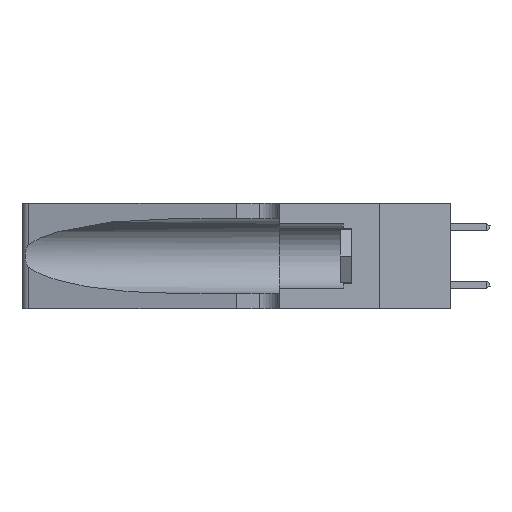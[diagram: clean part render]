
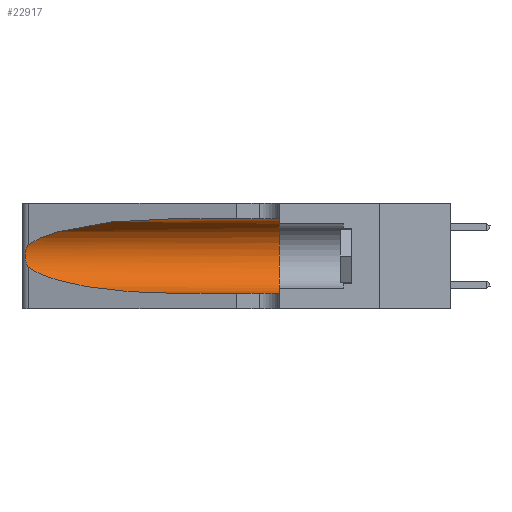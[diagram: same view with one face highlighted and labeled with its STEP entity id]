
A CAD part, left-side view. The second image highlights one B-rep face of the part: STEP entity #22917.
In plain terms, the highlighted cylindrical face has radius 3.308 mm (diameter 6.617 mm), a partial arc.
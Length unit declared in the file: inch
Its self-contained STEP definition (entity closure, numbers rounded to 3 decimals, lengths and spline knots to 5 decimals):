
#261 = AXIS2_PLACEMENT_3D ( 'NONE', #25124, #6758, #11429 ) ;
#1364 = DIRECTION ( 'NONE',  ( 0., -1., 0. ) ) ;
#1987 = CARTESIAN_POINT ( 'NONE',  ( 0.25487, 1.22718, 0.14631 ) ) ;
#2137 = CARTESIAN_POINT ( 'NONE',  ( 0.25639, 1.23184, 0.21858 ) ) ;
#2573 = ORIENTED_EDGE ( 'NONE', *, *, #3771, .T. ) ;
#2584 = CARTESIAN_POINT ( 'NONE',  ( 0.1305, 0.35, 0.05475 ) ) ;
#3664 = VERTEX_POINT ( 'NONE', #27870 ) ;
#3771 = EDGE_CURVE ( 'NONE', #14940, #25834, #26094, .T. ) ;
#3923 = CARTESIAN_POINT ( 'NONE',  ( 0.25487, 1.22718, 0.14631 ) ) ;
#4180 = AXIS2_PLACEMENT_3D ( 'NONE', #6070, #22220, #8388 ) ;
#4479 = CARTESIAN_POINT ( 'NONE',  ( 0.25854, 1.2359, 0.20912 ) ) ;
#4902 = CYLINDRICAL_SURFACE ( 'NONE', #261, 0.13025 ) ;
#5073 = CIRCLE ( 'NONE', #4180, 0.13025 ) ;
#5121 = CARTESIAN_POINT ( 'NONE',  ( 0.18966, 0.96281, 0.31525 ) ) ;
#5540 = ORIENTED_EDGE ( 'NONE', *, *, #24646, .F. ) ;
#6070 = CARTESIAN_POINT ( 'NONE',  ( 0.1305, 0.35, 0.185 ) ) ;
#6091 = B_SPLINE_CURVE_WITH_KNOTS ( 'NONE', 3,
 ( #25230, #13781, #2137, #18386, #4479, #20699, #6861, #23013, #9196, #25334, #11536, #27645, #13876, #29940 ),
 .UNSPECIFIED., .F., .F.,
 ( 4, 2, 2, 2, 2, 2, 4 ),
 ( 0., 0.00027, 0.00053, 0.00107, 0.0016, 0.00187, 0.00214 ),
 .UNSPECIFIED. ) ;
#6699 = EDGE_LOOP ( 'NONE', ( #2573, #14979, #21804, #27936, #10268, #5540 ) ) ;
#6758 = DIRECTION ( 'NONE',  ( 0., -1., 0. ) ) ;
#6861 = CARTESIAN_POINT ( 'NONE',  ( 0.26075, 1.23896, 0.19203 ) ) ;
#7002 = VECTOR ( 'NONE', #1364, 39.37008 ) ;
#8388 = DIRECTION ( 'NONE',  ( 0., 0., 1. ) ) ;
#8605 = VECTOR ( 'NONE', #23226, 39.37008 ) ;
#9196 = CARTESIAN_POINT ( 'NONE',  ( 0.26017, 1.23833, 0.17102 ) ) ;
#9337 = LINE ( 'NONE', #11652, #8605 ) ;
#9818 = CARTESIAN_POINT ( 'NONE',  ( 0.25487, 1.22718, 0.22369 ) ) ;
#10268 = ORIENTED_EDGE ( 'NONE', *, *, #13147, .F. ) ;
#11429 = DIRECTION ( 'NONE',  ( 0., 0., -1. ) ) ;
#11536 = CARTESIAN_POINT ( 'NONE',  ( 0.25789, 1.23486, 0.15765 ) ) ;
#11652 = CARTESIAN_POINT ( 'NONE',  ( 0.1305, 1.61858, 0.05475 ) ) ;
#12064 = CARTESIAN_POINT ( 'NONE',  ( 0.2373, 1.15595, 0.28018 ) ) ;
#12379 = CARTESIAN_POINT ( 'NONE',  ( 0.1305, 0.72297, 0.31525 ) ) ;
#13147 = EDGE_CURVE ( 'NONE', #3664, #26229, #5073, .T. ) ;
#13216 = CARTESIAN_POINT ( 'NONE',  ( 0.1305, 0.72297, 0.05475 ) ) ;
#13353 = EDGE_CURVE ( 'NONE', #25834, #23560, #6091, .T. ) ;
#13781 = CARTESIAN_POINT ( 'NONE',  ( 0.25555, 1.22994, 0.2215 ) ) ;
#13876 = CARTESIAN_POINT ( 'NONE',  ( 0.25555, 1.22993, 0.14849 ) ) ;
#14471 = VERTEX_POINT ( 'NONE', #13216 ) ;
#14940 = VERTEX_POINT ( 'NONE', #12379 ) ;
#14979 = ORIENTED_EDGE ( 'NONE', *, *, #13353, .T. ) ;
#15537 = CARTESIAN_POINT ( 'NONE',  ( 0.2373, 1.15595, 0.08982 ) ) ;
#15634 = CARTESIAN_POINT ( 'NONE',  ( 0.1305, 0.72297, 0.05475 ) ) ;
#18386 = CARTESIAN_POINT ( 'NONE',  ( 0.25787, 1.23484, 0.2124 ) ) ;
#19450 = CARTESIAN_POINT ( 'NONE',  ( 0.25487, 1.22718, 0.22369 ) ) ;
#20699 = CARTESIAN_POINT ( 'NONE',  ( 0.26018, 1.23835, 0.19895 ) ) ;
#21577 = EDGE_CURVE ( 'NONE', #23560, #14471, #28286, .T. ) ;
#21804 = ORIENTED_EDGE ( 'NONE', *, *, #21577, .T. ) ;
#22220 = DIRECTION ( 'NONE',  ( 0., 1., 0. ) ) ;
#22361 = EDGE_CURVE ( 'NONE', #14471, #26229, #9337, .T. ) ;
#22917 = ADVANCED_FACE ( 'NONE', ( #23356 ), #4902, .F. ) ;
#23013 = CARTESIAN_POINT ( 'NONE',  ( 0.26075, 1.23896, 0.178 ) ) ;
#23226 = DIRECTION ( 'NONE',  ( 0., -1., 0. ) ) ;
#23356 = FACE_OUTER_BOUND ( 'NONE', #6699, .T. ) ;
#23560 = VERTEX_POINT ( 'NONE', #1987 ) ;
#23621 = CARTESIAN_POINT ( 'NONE',  ( 0.1305, 0.72297, 0.31525 ) ) ;
#24646 = EDGE_CURVE ( 'NONE', #14940, #3664, #26139, .T. ) ;
#25124 = CARTESIAN_POINT ( 'NONE',  ( 0.1305, 1.61858, 0.185 ) ) ;
#25230 = CARTESIAN_POINT ( 'NONE',  ( 0.25487, 1.22718, 0.22369 ) ) ;
#25334 = CARTESIAN_POINT ( 'NONE',  ( 0.25856, 1.23593, 0.16098 ) ) ;
#25834 = VERTEX_POINT ( 'NONE', #19450 ) ;
#26094 =( BOUNDED_CURVE ( )  B_SPLINE_CURVE ( 3, ( #23621, #5121, #12064, #9818 ),
 .UNSPECIFIED., .F., .F. ) 
 B_SPLINE_CURVE_WITH_KNOTS ( ( 4, 4 ),
 ( 1.5708, 2.84003 ),
 .UNSPECIFIED. ) 
 CURVE ( )  GEOMETRIC_REPRESENTATION_ITEM ( )  RATIONAL_B_SPLINE_CURVE ( ( 1., 0.87, 0.87, 1. ) ) 
 REPRESENTATION_ITEM ( '' )  );
#26139 = LINE ( 'NONE', #28550, #7002 ) ;
#26229 = VERTEX_POINT ( 'NONE', #2584 ) ;
#27645 = CARTESIAN_POINT ( 'NONE',  ( 0.25639, 1.23186, 0.15144 ) ) ;
#27870 = CARTESIAN_POINT ( 'NONE',  ( 0.1305, 0.35, 0.31525 ) ) ;
#27936 = ORIENTED_EDGE ( 'NONE', *, *, #22361, .T. ) ;
#28286 =( BOUNDED_CURVE ( )  B_SPLINE_CURVE ( 3, ( #3923, #15537, #29387, #15634 ),
 .UNSPECIFIED., .F., .T. ) 
 B_SPLINE_CURVE_WITH_KNOTS ( ( 4, 4 ),
 ( 3.44316, 4.71239 ),
 .UNSPECIFIED. ) 
 CURVE ( )  GEOMETRIC_REPRESENTATION_ITEM ( )  RATIONAL_B_SPLINE_CURVE ( ( 1., 0.87, 0.87, 1. ) ) 
 REPRESENTATION_ITEM ( '' )  );
#28550 = CARTESIAN_POINT ( 'NONE',  ( 0.1305, 1.61858, 0.31525 ) ) ;
#29387 = CARTESIAN_POINT ( 'NONE',  ( 0.18966, 0.96281, 0.05475 ) ) ;
#29940 = CARTESIAN_POINT ( 'NONE',  ( 0.25487, 1.22718, 0.14631 ) ) ;
